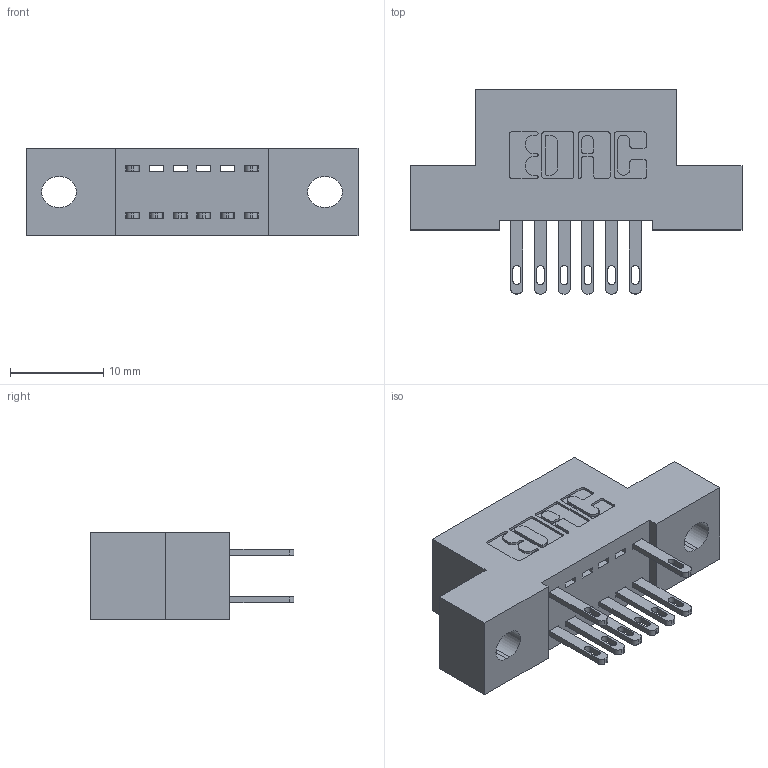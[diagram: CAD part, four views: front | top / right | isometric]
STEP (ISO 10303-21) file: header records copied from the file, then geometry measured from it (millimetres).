
FILE_DESCRIPTION (( 'STEP AP203' ), '1' );
FILE_NAME ('342-012-500-202.STEP', '2018-08-10T14:48:34', ( '' ), ( '' ), 'SwSTEP 2.0', 'SolidWorks 2016', '' );
FILE_SCHEMA (( 'CONFIG_CONTROL_DESIGN' ));
Length unit declared in the file: inch
Products named in the file (3): 342 Part_.128 Slot; 345-292-001_345-293-100; 342-012-500-202
Assembly tree (9 placements, depth 2):
  342-012-500-202
    342 Part_.128 Slot
    345-292-001_345-293-100  x8
Bounding box: 35.56 x 21.85 x 9.4 mm (x, y, z)
Volume: 2961 mm3; surface area: 3569.8 mm2
Topology: 9 solids, 9 shells, 522 faces, 1571 edges, 1046 vertices
Faces by surface type: plane 334, cylinder 188
Entity records: 8321 total; most frequent: CARTESIAN_POINT 1438, ORIENTED_EDGE 1378, DIRECTION 1289, EDGE_CURVE 689, VECTOR 557, LINE 557, VERTEX_POINT 458, AXIS2_PLACEMENT_3D 366
